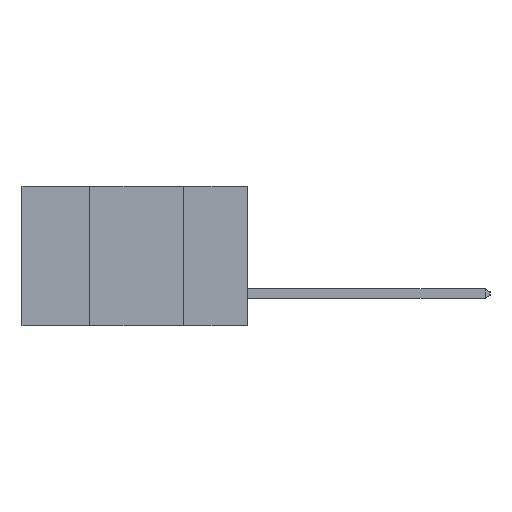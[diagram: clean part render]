
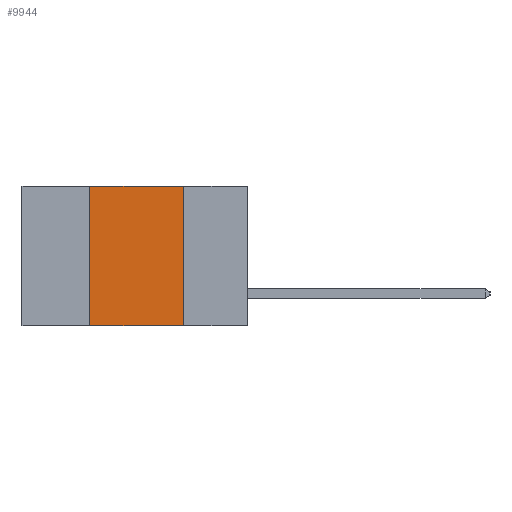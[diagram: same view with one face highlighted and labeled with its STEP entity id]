
A CAD part, left-side view. The second image highlights one B-rep face of the part: STEP entity #9944.
In plain terms, the highlighted planar face has unit normal (-1, 0, 0).
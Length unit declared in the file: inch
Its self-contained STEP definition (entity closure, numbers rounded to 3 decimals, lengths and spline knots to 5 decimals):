
#947 = LINE ( 'NONE', #28726, #13496 ) ;
#1266 = CARTESIAN_POINT ( 'NONE',  ( 0., 0.42, -0.37 ) ) ;
#2892 = EDGE_CURVE ( 'NONE', #19242, #9608, #28393, .T. ) ;
#3552 = VECTOR ( 'NONE', #14868, 39.37008 ) ;
#3890 = EDGE_LOOP ( 'NONE', ( #20768, #18145, #11077, #4428 ) ) ;
#4087 = DIRECTION ( 'NONE',  ( 0., -1., 0. ) ) ;
#4428 = ORIENTED_EDGE ( 'NONE', *, *, #31602, .T. ) ;
#6299 = CARTESIAN_POINT ( 'NONE',  ( 0., 0.42, 0. ) ) ;
#6603 = VERTEX_POINT ( 'NONE', #25682 ) ;
#7813 = PLANE ( 'NONE',  #12867 ) ;
#7901 = EDGE_CURVE ( 'NONE', #6603, #29689, #23656, .T. ) ;
#8152 = CARTESIAN_POINT ( 'NONE',  ( 0., 0.17, 0. ) ) ;
#8258 = DIRECTION ( 'NONE',  ( 0., 0., -1. ) ) ;
#9608 = VERTEX_POINT ( 'NONE', #6299 ) ;
#9688 = CARTESIAN_POINT ( 'NONE',  ( 0., 0.6, 0. ) ) ;
#9944 = ADVANCED_FACE ( 'NONE', ( #31175 ), #7813, .F. ) ;
#10350 = CARTESIAN_POINT ( 'NONE',  ( 0., 0.6, 0. ) ) ;
#10978 = LINE ( 'NONE', #9688, #3552 ) ;
#11077 = ORIENTED_EDGE ( 'NONE', *, *, #2892, .F. ) ;
#12866 = DIRECTION ( 'NONE',  ( 1., 0., 0. ) ) ;
#12867 = AXIS2_PLACEMENT_3D ( 'NONE', #10350, #12866, #30014 ) ;
#13496 = VECTOR ( 'NONE', #4087, 39.37008 ) ;
#14868 = DIRECTION ( 'NONE',  ( 0., -1., 0. ) ) ;
#16845 = CARTESIAN_POINT ( 'NONE',  ( 0., 0.17, -0.37 ) ) ;
#18145 = ORIENTED_EDGE ( 'NONE', *, *, #28797, .F. ) ;
#18990 = CARTESIAN_POINT ( 'NONE',  ( 0., 0.42, 0. ) ) ;
#19242 = VERTEX_POINT ( 'NONE', #1266 ) ;
#20768 = ORIENTED_EDGE ( 'NONE', *, *, #7901, .F. ) ;
#21917 = VECTOR ( 'NONE', #30401, 39.37008 ) ;
#23656 = LINE ( 'NONE', #8152, #27118 ) ;
#25682 = CARTESIAN_POINT ( 'NONE',  ( 0., 0.17, 0. ) ) ;
#27118 = VECTOR ( 'NONE', #8258, 39.37008 ) ;
#28393 = LINE ( 'NONE', #18990, #21917 ) ;
#28726 = CARTESIAN_POINT ( 'NONE',  ( 0., 0.6, -0.37 ) ) ;
#28797 = EDGE_CURVE ( 'NONE', #9608, #6603, #10978, .T. ) ;
#29689 = VERTEX_POINT ( 'NONE', #16845 ) ;
#30014 = DIRECTION ( 'NONE',  ( 0., 0., -1. ) ) ;
#30401 = DIRECTION ( 'NONE',  ( 0., 0., 1. ) ) ;
#31175 = FACE_OUTER_BOUND ( 'NONE', #3890, .T. ) ;
#31602 = EDGE_CURVE ( 'NONE', #19242, #29689, #947, .T. ) ;
